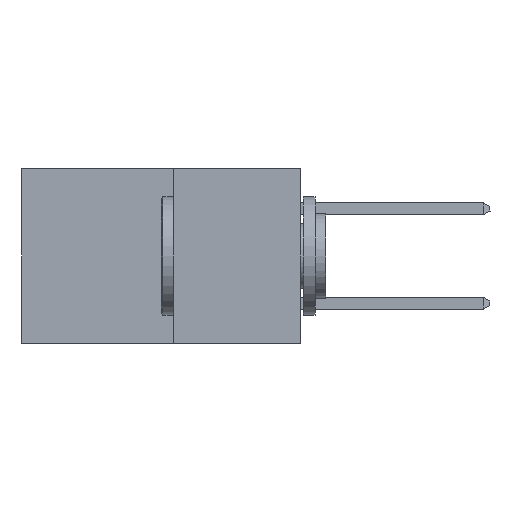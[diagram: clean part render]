
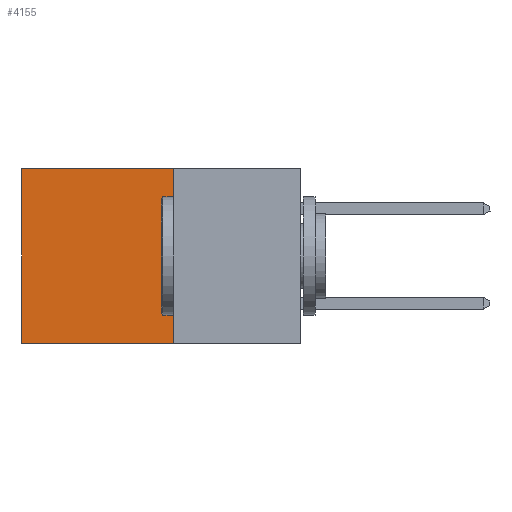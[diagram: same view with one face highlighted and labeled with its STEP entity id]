
A CAD part, left-side view. The second image highlights one B-rep face of the part: STEP entity #4155.
In plain terms, the highlighted planar face has unit normal (-1, 0, 0).
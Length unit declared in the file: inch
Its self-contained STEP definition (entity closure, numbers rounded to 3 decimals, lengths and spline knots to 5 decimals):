
#68 = LINE ( 'NONE', #1174, #12009 ) ;
#94 = CARTESIAN_POINT ( 'NONE',  ( 0.277, 0.27, 0. ) ) ;
#829 = LINE ( 'NONE', #94, #17208 ) ;
#1174 = CARTESIAN_POINT ( 'NONE',  ( 0.277, 0.27, -0.37 ) ) ;
#1721 = EDGE_CURVE ( 'NONE', #12088, #16363, #13436, .T. ) ;
#2130 = VERTEX_POINT ( 'NONE', #17034 ) ;
#2835 = EDGE_LOOP ( 'NONE', ( #16077, #14747, #10499, #17348 ) ) ;
#2916 = CARTESIAN_POINT ( 'NONE',  ( 0.277, 0.27, -0.37 ) ) ;
#4053 = CARTESIAN_POINT ( 'NONE',  ( 0.277, 0.27, -0.37 ) ) ;
#4155 = ADVANCED_FACE ( 'NONE', ( #17150 ), #5838, .F. ) ;
#4463 = DIRECTION ( 'NONE',  ( 0., 1., 0. ) ) ;
#5838 = PLANE ( 'NONE',  #11570 ) ;
#6506 = DIRECTION ( 'NONE',  ( 0., 0., -1. ) ) ;
#7235 = CARTESIAN_POINT ( 'NONE',  ( 0.277, 0.59, -0.37 ) ) ;
#7431 = DIRECTION ( 'NONE',  ( 0., 0., -1. ) ) ;
#7794 = CARTESIAN_POINT ( 'NONE',  ( 0.277, 0.27, -0.37 ) ) ;
#8133 = LINE ( 'NONE', #4053, #15566 ) ;
#8349 = CARTESIAN_POINT ( 'NONE',  ( 0.277, 0.59, 0. ) ) ;
#9516 = VECTOR ( 'NONE', #6506, 39.37008 ) ;
#10499 = ORIENTED_EDGE ( 'NONE', *, *, #18143, .F. ) ;
#11570 = AXIS2_PLACEMENT_3D ( 'NONE', #2916, #16333, #7431 ) ;
#12009 = VECTOR ( 'NONE', #4463, 39.37008 ) ;
#12075 = DIRECTION ( 'NONE',  ( 0., 1., 0. ) ) ;
#12088 = VERTEX_POINT ( 'NONE', #8349 ) ;
#13120 = EDGE_CURVE ( 'NONE', #2130, #12088, #829, .T. ) ;
#13436 = LINE ( 'NONE', #7235, #9516 ) ;
#14225 = EDGE_CURVE ( 'NONE', #15082, #16363, #68, .T. ) ;
#14747 = ORIENTED_EDGE ( 'NONE', *, *, #14225, .F. ) ;
#15082 = VERTEX_POINT ( 'NONE', #7794 ) ;
#15566 = VECTOR ( 'NONE', #15997, 39.37008 ) ;
#15997 = DIRECTION ( 'NONE',  ( 0., 0., -1. ) ) ;
#16077 = ORIENTED_EDGE ( 'NONE', *, *, #1721, .T. ) ;
#16333 = DIRECTION ( 'NONE',  ( 1., 0., 0. ) ) ;
#16363 = VERTEX_POINT ( 'NONE', #19253 ) ;
#17034 = CARTESIAN_POINT ( 'NONE',  ( 0.277, 0.27, 0. ) ) ;
#17150 = FACE_OUTER_BOUND ( 'NONE', #2835, .T. ) ;
#17208 = VECTOR ( 'NONE', #12075, 39.37008 ) ;
#17348 = ORIENTED_EDGE ( 'NONE', *, *, #13120, .T. ) ;
#18143 = EDGE_CURVE ( 'NONE', #2130, #15082, #8133, .T. ) ;
#19253 = CARTESIAN_POINT ( 'NONE',  ( 0.277, 0.59, -0.37 ) ) ;
